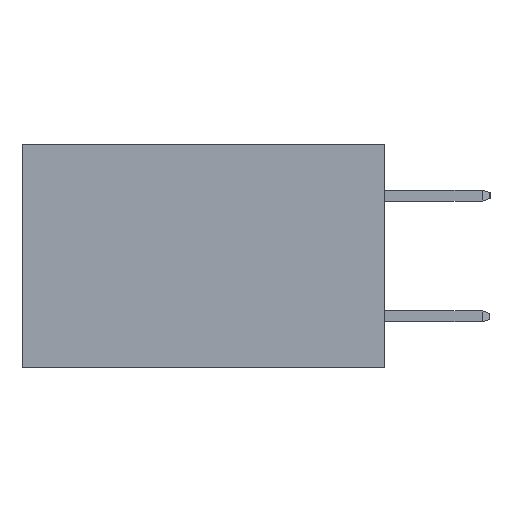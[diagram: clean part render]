
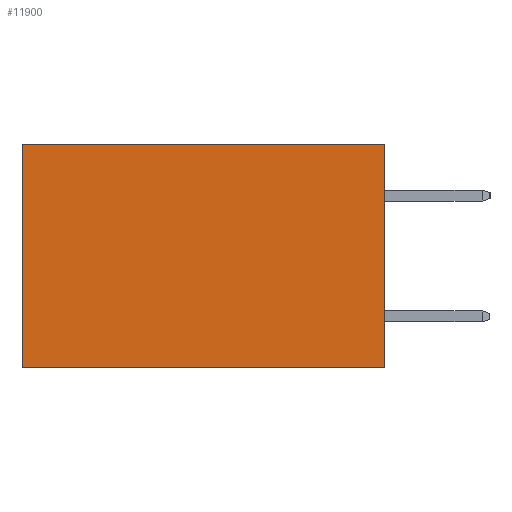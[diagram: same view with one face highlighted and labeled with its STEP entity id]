
A CAD part, left-side view. The second image highlights one B-rep face of the part: STEP entity #11900.
In plain terms, the highlighted planar face has unit normal (-1, 0, 0).
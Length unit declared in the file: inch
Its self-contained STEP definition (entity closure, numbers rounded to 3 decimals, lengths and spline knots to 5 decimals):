
#364 = CARTESIAN_POINT ( 'NONE',  ( 0.298, 0., -0.37 ) ) ;
#814 = DIRECTION ( 'NONE',  ( 0., 0., -1. ) ) ;
#844 = EDGE_CURVE ( 'NONE', #1613, #7486, #19024, .T. ) ;
#1537 = DIRECTION ( 'NONE',  ( 0., 1., 0. ) ) ;
#1613 = VERTEX_POINT ( 'NONE', #15690 ) ;
#2081 = CARTESIAN_POINT ( 'NONE',  ( 0.298, 0.6, 0. ) ) ;
#2098 = VERTEX_POINT ( 'NONE', #8578 ) ;
#2319 = VECTOR ( 'NONE', #8463, 39.37008 ) ;
#3776 = VECTOR ( 'NONE', #11756, 39.37008 ) ;
#4545 = VECTOR ( 'NONE', #6538, 39.37008 ) ;
#6538 = DIRECTION ( 'NONE',  ( 0., 0., -1. ) ) ;
#7017 = CARTESIAN_POINT ( 'NONE',  ( 0.298, 0., 0. ) ) ;
#7018 = VECTOR ( 'NONE', #1537, 39.37008 ) ;
#7486 = VERTEX_POINT ( 'NONE', #13566 ) ;
#8410 = AXIS2_PLACEMENT_3D ( 'NONE', #14322, #9789, #814 ) ;
#8463 = DIRECTION ( 'NONE',  ( 0., 1., 0. ) ) ;
#8578 = CARTESIAN_POINT ( 'NONE',  ( 0.298, 0.6, 0. ) ) ;
#9789 = DIRECTION ( 'NONE',  ( 1., 0., 0. ) ) ;
#10919 = ORIENTED_EDGE ( 'NONE', *, *, #11974, .T. ) ;
#11693 = FACE_OUTER_BOUND ( 'NONE', #11815, .T. ) ;
#11749 = LINE ( 'NONE', #16274, #3776 ) ;
#11756 = DIRECTION ( 'NONE',  ( 0., 0., -1. ) ) ;
#11815 = EDGE_LOOP ( 'NONE', ( #17995, #16387, #16865, #10919 ) ) ;
#11900 = ADVANCED_FACE ( 'NONE', ( #11693 ), #18802, .F. ) ;
#11974 = EDGE_CURVE ( 'NONE', #15983, #2098, #14303, .T. ) ;
#13566 = CARTESIAN_POINT ( 'NONE',  ( 0.298, 0.6, -0.37 ) ) ;
#14303 = LINE ( 'NONE', #16048, #2319 ) ;
#14322 = CARTESIAN_POINT ( 'NONE',  ( 0.298, 0., 0. ) ) ;
#14575 = EDGE_CURVE ( 'NONE', #2098, #7486, #16561, .T. ) ;
#15690 = CARTESIAN_POINT ( 'NONE',  ( 0.298, 0., -0.37 ) ) ;
#15983 = VERTEX_POINT ( 'NONE', #7017 ) ;
#16048 = CARTESIAN_POINT ( 'NONE',  ( 0.298, 0., 0. ) ) ;
#16274 = CARTESIAN_POINT ( 'NONE',  ( 0.298, 0., 0. ) ) ;
#16387 = ORIENTED_EDGE ( 'NONE', *, *, #844, .F. ) ;
#16561 = LINE ( 'NONE', #2081, #4545 ) ;
#16865 = ORIENTED_EDGE ( 'NONE', *, *, #17317, .F. ) ;
#17317 = EDGE_CURVE ( 'NONE', #15983, #1613, #11749, .T. ) ;
#17995 = ORIENTED_EDGE ( 'NONE', *, *, #14575, .T. ) ;
#18802 = PLANE ( 'NONE',  #8410 ) ;
#19024 = LINE ( 'NONE', #364, #7018 ) ;
